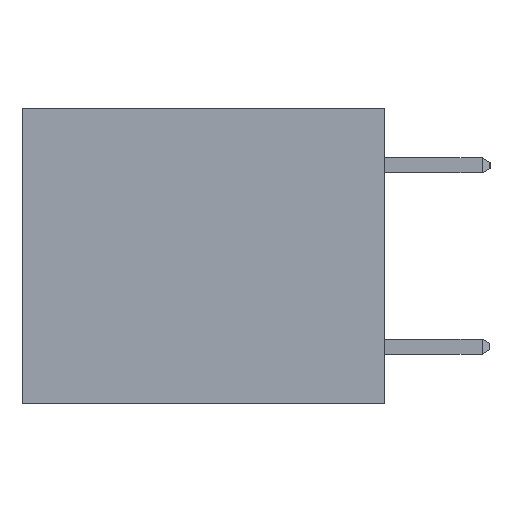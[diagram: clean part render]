
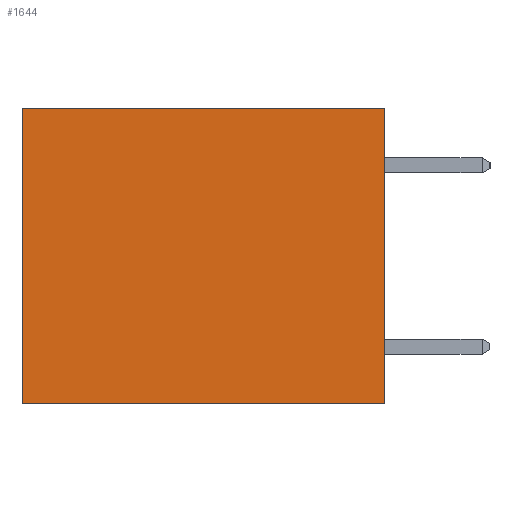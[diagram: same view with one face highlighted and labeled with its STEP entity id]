
A CAD part, left-side view. The second image highlights one B-rep face of the part: STEP entity #1644.
In plain terms, the highlighted planar face has unit normal (-1, 0, 0).
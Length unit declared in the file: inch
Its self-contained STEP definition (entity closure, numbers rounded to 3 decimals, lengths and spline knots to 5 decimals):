
#686 = ORIENTED_EDGE ( 'NONE', *, *, #15242, .F. ) ;
#801 = PLANE ( 'NONE',  #13412 ) ;
#1092 = VERTEX_POINT ( 'NONE', #13778 ) ;
#1644 = ADVANCED_FACE ( 'NONE', ( #11369 ), #801, .F. ) ;
#1778 = VECTOR ( 'NONE', #2306, 39.37008 ) ;
#1953 = DIRECTION ( 'NONE',  ( 0., 1., 0. ) ) ;
#1984 = VERTEX_POINT ( 'NONE', #6698 ) ;
#2306 = DIRECTION ( 'NONE',  ( 0., 0., -1. ) ) ;
#3000 = EDGE_CURVE ( 'NONE', #1984, #8725, #14856, .T. ) ;
#3766 = CARTESIAN_POINT ( 'NONE',  ( 0.3165, 0.6, -0.49 ) ) ;
#3918 = CARTESIAN_POINT ( 'NONE',  ( 0.3165, 0., -0.49 ) ) ;
#4170 = CARTESIAN_POINT ( 'NONE',  ( 0.3165, 0.6, -0.49 ) ) ;
#5605 = VECTOR ( 'NONE', #8392, 39.37008 ) ;
#6698 = CARTESIAN_POINT ( 'NONE',  ( 0.3165, 0.6, 0. ) ) ;
#6790 = VECTOR ( 'NONE', #16385, 39.37008 ) ;
#7280 = LINE ( 'NONE', #7937, #14631 ) ;
#7514 = LINE ( 'NONE', #17305, #1778 ) ;
#7572 = ORIENTED_EDGE ( 'NONE', *, *, #9721, .F. ) ;
#7937 = CARTESIAN_POINT ( 'NONE',  ( 0.3165, 0., -0.49 ) ) ;
#8392 = DIRECTION ( 'NONE',  ( 0., 1., 0. ) ) ;
#8725 = VERTEX_POINT ( 'NONE', #3766 ) ;
#9098 = ORIENTED_EDGE ( 'NONE', *, *, #3000, .T. ) ;
#9721 = EDGE_CURVE ( 'NONE', #10893, #8725, #7280, .T. ) ;
#9723 = DIRECTION ( 'NONE',  ( 1., 0., 0. ) ) ;
#10893 = VERTEX_POINT ( 'NONE', #3918 ) ;
#11369 = FACE_OUTER_BOUND ( 'NONE', #13626, .T. ) ;
#12402 = ORIENTED_EDGE ( 'NONE', *, *, #16159, .T. ) ;
#13412 = AXIS2_PLACEMENT_3D ( 'NONE', #17473, #9723, #18948 ) ;
#13626 = EDGE_LOOP ( 'NONE', ( #9098, #7572, #686, #12402 ) ) ;
#13778 = CARTESIAN_POINT ( 'NONE',  ( 0.3165, 0., 0. ) ) ;
#14631 = VECTOR ( 'NONE', #1953, 39.37008 ) ;
#14856 = LINE ( 'NONE', #4170, #6790 ) ;
#15242 = EDGE_CURVE ( 'NONE', #1092, #10893, #7514, .T. ) ;
#15839 = CARTESIAN_POINT ( 'NONE',  ( 0.3165, 0., 0. ) ) ;
#16056 = LINE ( 'NONE', #15839, #5605 ) ;
#16159 = EDGE_CURVE ( 'NONE', #1092, #1984, #16056, .T. ) ;
#16385 = DIRECTION ( 'NONE',  ( 0., 0., -1. ) ) ;
#17305 = CARTESIAN_POINT ( 'NONE',  ( 0.3165, 0., -0.49 ) ) ;
#17473 = CARTESIAN_POINT ( 'NONE',  ( 0.3165, 0., -0.49 ) ) ;
#18948 = DIRECTION ( 'NONE',  ( 0., 0., -1. ) ) ;
